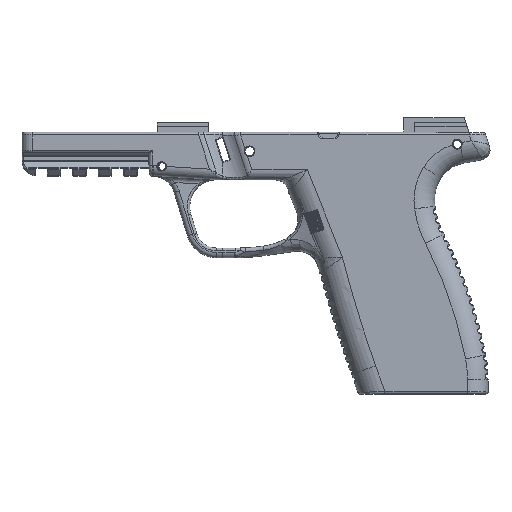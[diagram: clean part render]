
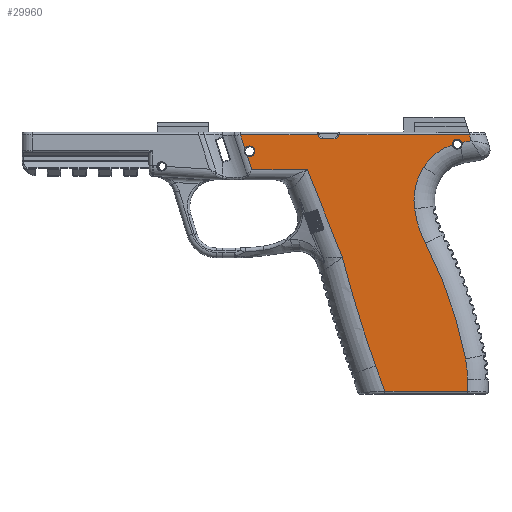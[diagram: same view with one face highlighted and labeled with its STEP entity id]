
A CAD part, top view. The second image highlights one B-rep face of the part: STEP entity #29960.
In plain terms, the highlighted planar face has unit normal (0, 0, 1).
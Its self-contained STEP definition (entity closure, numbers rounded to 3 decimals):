
#1770=ELLIPSE('',#32216,2.296,2.089);
#1771=ELLIPSE('',#32218,1.268,0.846);
#3258=CIRCLE('',#32207,1.5);
#3259=CIRCLE('',#32208,1.5);
#3260=CIRCLE('',#32209,2.05);
#3261=CIRCLE('',#32210,440.);
#3262=CIRCLE('',#32211,42.);
#3263=CIRCLE('',#32212,167.5);
#3264=CIRCLE('',#32213,42.121);
#3265=CIRCLE('',#32214,24.045);
#3266=CIRCLE('',#32215,21.06);
#3267=CIRCLE('',#32217,1.9);
#5002=FACE_OUTER_BOUND('',#6968,.T.);
#6968=EDGE_LOOP('',(#21092,#21093,#21094,#21095,#21096,#21097,#21098,#21099,
#21100,#21101,#21102,#21103,#21104,#21105,#21106,#21107,#21108,#21109,#21110,
#21111,#21112,#21113,#21114,#21115));
#9044=LINE('',#46971,#10744);
#9052=LINE('',#47210,#10752);
#9062=LINE('',#47299,#10762);
#9063=LINE('',#47304,#10763);
#9064=LINE('',#47306,#10764);
#9065=LINE('',#47308,#10765);
#9066=LINE('',#47312,#10766);
#9067=LINE('',#47316,#10767);
#9068=LINE('',#47318,#10768);
#9069=LINE('',#47322,#10769);
#9070=LINE('',#47323,#10770);
#9071=LINE('',#47326,#10771);
#10744=VECTOR('',#36630,10.);
#10752=VECTOR('',#36676,10.);
#10762=VECTOR('',#36698,10.);
#10763=VECTOR('',#36703,10.);
#10764=VECTOR('',#36704,10.);
#10765=VECTOR('',#36705,10.);
#10766=VECTOR('',#36708,10.);
#10767=VECTOR('',#36711,10.);
#10768=VECTOR('',#36712,10.);
#10769=VECTOR('',#36715,10.);
#10770=VECTOR('',#36716,10.);
#10771=VECTOR('',#36719,10.);
#12508=VERTEX_POINT('',#46961);
#12509=VERTEX_POINT('',#46970);
#12518=VERTEX_POINT('',#47031);
#12530=VERTEX_POINT('',#47208);
#12551=VERTEX_POINT('',#47298);
#12552=VERTEX_POINT('',#47302);
#12553=VERTEX_POINT('',#47303);
#12554=VERTEX_POINT('',#47305);
#12555=VERTEX_POINT('',#47307);
#12556=VERTEX_POINT('',#47309);
#12557=VERTEX_POINT('',#47311);
#12558=VERTEX_POINT('',#47313);
#12559=VERTEX_POINT('',#47315);
#12560=VERTEX_POINT('',#47317);
#12561=VERTEX_POINT('',#47319);
#12562=VERTEX_POINT('',#47321);
#12563=VERTEX_POINT('',#47324);
#12564=VERTEX_POINT('',#47327);
#12565=VERTEX_POINT('',#47329);
#12566=VERTEX_POINT('',#47331);
#12567=VERTEX_POINT('',#47333);
#12568=VERTEX_POINT('',#47335);
#12569=VERTEX_POINT('',#47337);
#12570=VERTEX_POINT('',#47339);
#15607=EDGE_CURVE('',#12508,#12509,#9044,.T.);
#15635=EDGE_CURVE('',#12530,#12518,#9052,.T.);
#15657=EDGE_CURVE('',#12518,#12551,#9062,.T.);
#15659=EDGE_CURVE('',#12552,#12553,#9063,.T.);
#15660=EDGE_CURVE('',#12554,#12552,#9064,.T.);
#15661=EDGE_CURVE('',#12555,#12554,#9065,.T.);
#15662=EDGE_CURVE('',#12556,#12555,#3258,.T.);
#15663=EDGE_CURVE('',#12557,#12556,#9066,.T.);
#15664=EDGE_CURVE('',#12558,#12557,#3259,.T.);
#15665=EDGE_CURVE('',#12559,#12558,#9067,.T.);
#15666=EDGE_CURVE('',#12560,#12559,#9068,.T.);
#15667=EDGE_CURVE('',#12561,#12560,#3260,.T.);
#15668=EDGE_CURVE('',#12562,#12561,#9069,.T.);
#15669=EDGE_CURVE('',#12509,#12562,#9070,.T.);
#15670=EDGE_CURVE('',#12563,#12508,#3261,.T.);
#15671=EDGE_CURVE('',#12551,#12563,#9071,.T.);
#15672=EDGE_CURVE('',#12564,#12530,#3262,.T.);
#15673=EDGE_CURVE('',#12565,#12564,#3263,.T.);
#15674=EDGE_CURVE('',#12566,#12565,#3264,.T.);
#15675=EDGE_CURVE('',#12567,#12566,#3265,.T.);
#15676=EDGE_CURVE('',#12568,#12567,#3266,.T.);
#15677=EDGE_CURVE('',#12569,#12568,#1770,.T.);
#15678=EDGE_CURVE('',#12570,#12569,#3267,.T.);
#15679=EDGE_CURVE('',#12553,#12570,#1771,.T.);
#21092=ORIENTED_EDGE('',*,*,#15659,.F.);
#21093=ORIENTED_EDGE('',*,*,#15660,.F.);
#21094=ORIENTED_EDGE('',*,*,#15661,.F.);
#21095=ORIENTED_EDGE('',*,*,#15662,.F.);
#21096=ORIENTED_EDGE('',*,*,#15663,.F.);
#21097=ORIENTED_EDGE('',*,*,#15664,.F.);
#21098=ORIENTED_EDGE('',*,*,#15665,.F.);
#21099=ORIENTED_EDGE('',*,*,#15666,.F.);
#21100=ORIENTED_EDGE('',*,*,#15667,.F.);
#21101=ORIENTED_EDGE('',*,*,#15668,.F.);
#21102=ORIENTED_EDGE('',*,*,#15669,.F.);
#21103=ORIENTED_EDGE('',*,*,#15607,.F.);
#21104=ORIENTED_EDGE('',*,*,#15670,.F.);
#21105=ORIENTED_EDGE('',*,*,#15671,.F.);
#21106=ORIENTED_EDGE('',*,*,#15657,.F.);
#21107=ORIENTED_EDGE('',*,*,#15635,.F.);
#21108=ORIENTED_EDGE('',*,*,#15672,.F.);
#21109=ORIENTED_EDGE('',*,*,#15673,.F.);
#21110=ORIENTED_EDGE('',*,*,#15674,.F.);
#21111=ORIENTED_EDGE('',*,*,#15675,.F.);
#21112=ORIENTED_EDGE('',*,*,#15676,.F.);
#21113=ORIENTED_EDGE('',*,*,#15677,.F.);
#21114=ORIENTED_EDGE('',*,*,#15678,.F.);
#21115=ORIENTED_EDGE('',*,*,#15679,.F.);
#29385=PLANE('',#32206);
#29960=ADVANCED_FACE('',(#5002),#29385,.T.);
#32206=AXIS2_PLACEMENT_3D('',#47301,#36701,#36702);
#32207=AXIS2_PLACEMENT_3D('',#47310,#36706,#36707);
#32208=AXIS2_PLACEMENT_3D('',#47314,#36709,#36710);
#32209=AXIS2_PLACEMENT_3D('',#47320,#36713,#36714);
#32210=AXIS2_PLACEMENT_3D('',#47325,#36717,#36718);
#32211=AXIS2_PLACEMENT_3D('',#47328,#36720,#36721);
#32212=AXIS2_PLACEMENT_3D('',#47330,#36722,#36723);
#32213=AXIS2_PLACEMENT_3D('',#47332,#36724,#36725);
#32214=AXIS2_PLACEMENT_3D('',#47334,#36726,#36727);
#32215=AXIS2_PLACEMENT_3D('',#47336,#36728,#36729);
#32216=AXIS2_PLACEMENT_3D('',#47338,#36730,#36731);
#32217=AXIS2_PLACEMENT_3D('',#47340,#36732,#36733);
#32218=AXIS2_PLACEMENT_3D('',#47341,#36734,#36735);
#36630=DIRECTION('',(-0.371,0.929,0.));
#36676=DIRECTION('',(0.,-1.,0.));
#36698=DIRECTION('',(-1.,0.,0.));
#36701=DIRECTION('center_axis',(0.,0.,1.));
#36702=DIRECTION('ref_axis',(1.,0.,0.));
#36703=DIRECTION('',(-0.985,-0.174,0.));
#36704=DIRECTION('',(0.309,-0.951,0.));
#36705=DIRECTION('',(1.,0.,0.));
#36706=DIRECTION('center_axis',(0.,0.,1.));
#36707=DIRECTION('ref_axis',(0.707,-0.707,0.));
#36708=DIRECTION('',(1.,0.,0.));
#36709=DIRECTION('center_axis',(0.,0.,1.));
#36710=DIRECTION('ref_axis',(-0.707,-0.707,0.));
#36711=DIRECTION('',(1.,0.,0.));
#36712=DIRECTION('',(-0.309,0.951,0.));
#36713=DIRECTION('center_axis',(0.,0.,1.));
#36714=DIRECTION('ref_axis',(1.,0.,0.));
#36715=DIRECTION('',(-0.309,0.951,0.));
#36716=DIRECTION('',(-1.,0.,0.));
#36717=DIRECTION('center_axis',(0.,0.,-1.));
#36718=DIRECTION('ref_axis',(-0.956,-0.294,0.));
#36719=DIRECTION('',(-0.34,0.94,0.));
#36720=DIRECTION('center_axis',(0.,0.,-1.));
#36721=DIRECTION('ref_axis',(0.995,0.095,0.));
#36722=DIRECTION('center_axis',(0.,0.,-1.));
#36723=DIRECTION('ref_axis',(0.945,0.327,0.));
#36724=DIRECTION('center_axis',(0.,0.,1.));
#36725=DIRECTION('ref_axis',(-0.953,-0.303,0.));
#36726=DIRECTION('center_axis',(0.,0.,1.));
#36727=DIRECTION('ref_axis',(-0.978,0.21,0.));
#36728=DIRECTION('center_axis',(0.,0.,1.));
#36729=DIRECTION('ref_axis',(-0.557,0.83,0.));
#36730=DIRECTION('center_axis',(0.,0.,1.));
#36731=DIRECTION('ref_axis',(0.993,0.121,0.));
#36732=DIRECTION('center_axis',(0.,0.,1.));
#36733=DIRECTION('ref_axis',(-1.,0.,0.));
#36734=DIRECTION('center_axis',(0.,0.,1.));
#36735=DIRECTION('ref_axis',(0.358,-0.934,0.));
#46961=CARTESIAN_POINT('',(39.532,-4.905,13.5));
#46970=CARTESIAN_POINT('',(25.898,29.25,13.5));
#46971=CARTESIAN_POINT('',(37.534,0.1,13.5));
#47031=CARTESIAN_POINT('',(88.137,-57.,13.5));
#47208=CARTESIAN_POINT('',(88.137,-52.304,13.5));
#47210=CARTESIAN_POINT('',(88.137,-33.837,13.5));
#47298=CARTESIAN_POINT('',(56.053,-57.,13.5));
#47299=CARTESIAN_POINT('',(26.346,-57.,13.5));
#47301=CARTESIAN_POINT('Origin',(4.319,-9.978,13.5));
#47302=CARTESIAN_POINT('',(89.647,40.436,13.5));
#47303=CARTESIAN_POINT('',(85.91,39.777,13.5));
#47304=CARTESIAN_POINT('',(41.632,31.969,13.5));
#47305=CARTESIAN_POINT('',(88.895,42.75,13.5));
#47306=CARTESIAN_POINT('',(93.252,29.341,13.5));
#47307=CARTESIAN_POINT('',(38.15,42.75,13.5));
#47308=CARTESIAN_POINT('',(48.284,42.75,13.5));
#47309=CARTESIAN_POINT('',(36.65,41.25,13.5));
#47310=CARTESIAN_POINT('Origin',(36.65,42.75,13.5));
#47311=CARTESIAN_POINT('',(31.65,41.25,13.5));
#47312=CARTESIAN_POINT('',(20.984,41.25,13.5));
#47313=CARTESIAN_POINT('',(30.15,42.75,13.5));
#47314=CARTESIAN_POINT('Origin',(31.65,42.75,13.5));
#47315=CARTESIAN_POINT('',(-0.079,42.75,13.5));
#47316=CARTESIAN_POINT('',(48.284,42.75,13.5));
#47317=CARTESIAN_POINT('',(1.665,37.383,13.5));
#47318=CARTESIAN_POINT('',(2.358,35.25,13.5));
#47319=CARTESIAN_POINT('',(2.598,34.51,13.5));
#47320=CARTESIAN_POINT('Origin',(3.45,36.375,13.5));
#47321=CARTESIAN_POINT('',(4.307,29.25,13.5));
#47322=CARTESIAN_POINT('',(2.358,35.25,13.5));
#47323=CARTESIAN_POINT('',(7.909,29.25,13.5));
#47324=CARTESIAN_POINT('',(52.42,-46.966,13.5));
#47325=CARTESIAN_POINT('Origin',(466.143,102.814,13.5));
#47326=CARTESIAN_POINT('',(45.005,-26.484,13.5));
#47327=CARTESIAN_POINT('',(87.374,-44.334,13.5));
#47328=CARTESIAN_POINT('Origin',(46.137,-52.304,13.5));
#47329=CARTESIAN_POINT('',(71.832,0.566,13.5));
#47330=CARTESIAN_POINT('Origin',(-77.082,-76.119,13.5));
#47331=CARTESIAN_POINT('',(67.574,13.949,13.5));
#47332=CARTESIAN_POINT('Origin',(109.279,19.85,13.5));
#47333=CARTESIAN_POINT('',(71.05,30.155,13.5));
#47334=CARTESIAN_POINT('Origin',(91.382,17.318,13.5));
#47335=CARTESIAN_POINT('',(82.238,38.904,13.5));
#47336=CARTESIAN_POINT('Origin',(88.858,18.911,13.5));
#47337=CARTESIAN_POINT('',(82.232,38.962,13.5));
#47338=CARTESIAN_POINT('Origin',(84.518,39.173,13.5));
#47339=CARTESIAN_POINT('',(85.892,39.825,13.5));
#47340=CARTESIAN_POINT('Origin',(84.125,39.125,13.5));
#47341=CARTESIAN_POINT('Origin',(85.109,39.502,13.5));
